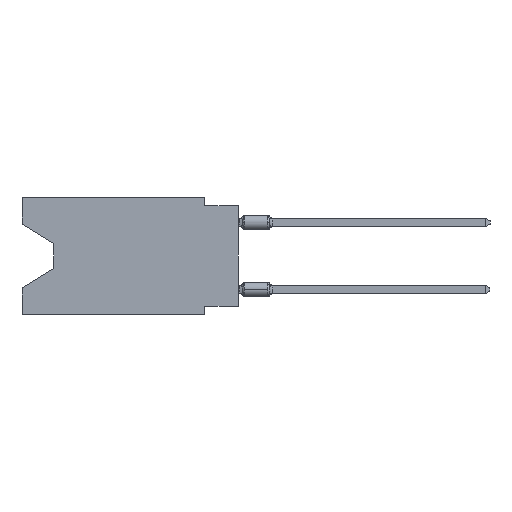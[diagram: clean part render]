
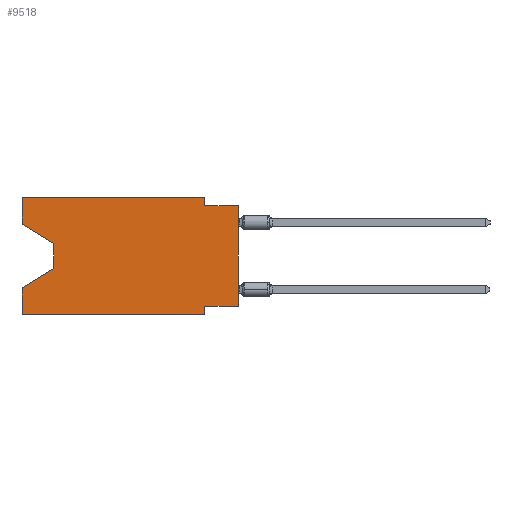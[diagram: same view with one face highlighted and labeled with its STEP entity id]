
A CAD part, left-side view. The second image highlights one B-rep face of the part: STEP entity #9518.
In plain terms, the highlighted planar face has unit normal (-1, 0, 0).
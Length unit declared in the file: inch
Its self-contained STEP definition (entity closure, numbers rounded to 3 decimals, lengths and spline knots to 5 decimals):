
#303 = CARTESIAN_POINT ( 'NONE',  ( 0., 0.55, -0.138 ) ) ;
#443 = EDGE_CURVE ( 'NONE', #11186, #7588, #18882, .T. ) ;
#929 = ORIENTED_EDGE ( 'NONE', *, *, #18731, .T. ) ;
#993 = VERTEX_POINT ( 'NONE', #1074 ) ;
#1074 = CARTESIAN_POINT ( 'NONE',  ( 0., 0.55, -0.212 ) ) ;
#1150 = DIRECTION ( 'NONE',  ( 0., 0., 1. ) ) ;
#1407 = LINE ( 'NONE', #15673, #16757 ) ;
#1430 = VERTEX_POINT ( 'NONE', #22394 ) ;
#1436 = AXIS2_PLACEMENT_3D ( 'NONE', #5542, #10573, #9273 ) ;
#1510 = EDGE_CURVE ( 'NONE', #8110, #21449, #4860, .T. ) ;
#1515 = CARTESIAN_POINT ( 'NONE',  ( 0., 0., -0.025 ) ) ;
#1518 = ORIENTED_EDGE ( 'NONE', *, *, #11480, .T. ) ;
#2066 = LINE ( 'NONE', #16099, #15612 ) ;
#2118 = VECTOR ( 'NONE', #10747, 39.37008 ) ;
#2246 = DIRECTION ( 'NONE',  ( 0., 0.855, -0.519 ) ) ;
#2607 = LINE ( 'NONE', #9733, #12410 ) ;
#2811 = DIRECTION ( 'NONE',  ( 0., 1., 0. ) ) ;
#3216 = CARTESIAN_POINT ( 'NONE',  ( 0., 0.1, 0. ) ) ;
#4379 = CARTESIAN_POINT ( 'NONE',  ( 0., 0.1, -0.325 ) ) ;
#4406 = ORIENTED_EDGE ( 'NONE', *, *, #1510, .F. ) ;
#4527 = ORIENTED_EDGE ( 'NONE', *, *, #6099, .T. ) ;
#4860 = LINE ( 'NONE', #3216, #6358 ) ;
#4877 = VERTEX_POINT ( 'NONE', #17801 ) ;
#4920 = ORIENTED_EDGE ( 'NONE', *, *, #9210, .F. ) ;
#5077 = CARTESIAN_POINT ( 'NONE',  ( 0., 0.1, -0.025 ) ) ;
#5542 = CARTESIAN_POINT ( 'NONE',  ( 0., 0.645, 0. ) ) ;
#6088 = LINE ( 'NONE', #10903, #22786 ) ;
#6099 = EDGE_CURVE ( 'NONE', #993, #4877, #6088, .T. ) ;
#6358 = VECTOR ( 'NONE', #14212, 39.37008 ) ;
#6396 = DIRECTION ( 'NONE',  ( 0., 0., -1. ) ) ;
#6989 = VECTOR ( 'NONE', #15302, 39.37008 ) ;
#7288 = CARTESIAN_POINT ( 'NONE',  ( 0., 0.645, -0.08025 ) ) ;
#7406 = FACE_OUTER_BOUND ( 'NONE', #14435, .T. ) ;
#7588 = VERTEX_POINT ( 'NONE', #12220 ) ;
#7986 = DIRECTION ( 'NONE',  ( 0., 0., 1. ) ) ;
#8110 = VERTEX_POINT ( 'NONE', #21863 ) ;
#8882 = ORIENTED_EDGE ( 'NONE', *, *, #16438, .F. ) ;
#9046 = PLANE ( 'NONE',  #1436 ) ;
#9210 = EDGE_CURVE ( 'NONE', #11186, #4877, #2066, .T. ) ;
#9273 = DIRECTION ( 'NONE',  ( 0., 0., -1. ) ) ;
#9518 = ADVANCED_FACE ( 'NONE', ( #7406 ), #9046, .F. ) ;
#9684 = ORIENTED_EDGE ( 'NONE', *, *, #15405, .F. ) ;
#9733 = CARTESIAN_POINT ( 'NONE',  ( 0., 0., 0. ) ) ;
#10573 = DIRECTION ( 'NONE',  ( 1., 0., 0. ) ) ;
#10747 = DIRECTION ( 'NONE',  ( 0., 0., -1. ) ) ;
#10903 = CARTESIAN_POINT ( 'NONE',  ( 0., 0.55, -0.212 ) ) ;
#11186 = VERTEX_POINT ( 'NONE', #22391 ) ;
#11480 = EDGE_CURVE ( 'NONE', #22761, #16186, #2607, .T. ) ;
#11852 = EDGE_CURVE ( 'NONE', #1430, #8110, #13432, .T. ) ;
#11907 = CARTESIAN_POINT ( 'NONE',  ( 0., 0.645, 0. ) ) ;
#12006 = DIRECTION ( 'NONE',  ( 0., -1., 0. ) ) ;
#12025 = CARTESIAN_POINT ( 'NONE',  ( 0., 0., -0.025 ) ) ;
#12220 = CARTESIAN_POINT ( 'NONE',  ( 0., 0.1, -0.35 ) ) ;
#12369 = ORIENTED_EDGE ( 'NONE', *, *, #17513, .T. ) ;
#12410 = VECTOR ( 'NONE', #7986, 39.37008 ) ;
#13432 = LINE ( 'NONE', #17173, #18746 ) ;
#13884 = CARTESIAN_POINT ( 'NONE',  ( 0., 0.645, -0.35 ) ) ;
#14148 = LINE ( 'NONE', #21262, #2118 ) ;
#14163 = EDGE_CURVE ( 'NONE', #21476, #1430, #17052, .T. ) ;
#14212 = DIRECTION ( 'NONE',  ( 0., 0., -1. ) ) ;
#14435 = EDGE_LOOP ( 'NONE', ( #929, #12369, #4527, #4920, #17405, #8882, #16247, #1518, #9684, #4406, #15905, #21854 ) ) ;
#15302 = DIRECTION ( 'NONE',  ( 0., -1., 0. ) ) ;
#15405 = EDGE_CURVE ( 'NONE', #21449, #16186, #22775, .T. ) ;
#15597 = VERTEX_POINT ( 'NONE', #303 ) ;
#15602 = VECTOR ( 'NONE', #12006, 39.37008 ) ;
#15612 = VECTOR ( 'NONE', #20049, 39.37008 ) ;
#15641 = LINE ( 'NONE', #22767, #23085 ) ;
#15673 = CARTESIAN_POINT ( 'NONE',  ( 0., 0., -0.325 ) ) ;
#15905 = ORIENTED_EDGE ( 'NONE', *, *, #11852, .F. ) ;
#16099 = CARTESIAN_POINT ( 'NONE',  ( 0., 0.645, 0. ) ) ;
#16186 = VERTEX_POINT ( 'NONE', #1515 ) ;
#16247 = ORIENTED_EDGE ( 'NONE', *, *, #17336, .F. ) ;
#16438 = EDGE_CURVE ( 'NONE', #17982, #7588, #15641, .T. ) ;
#16757 = VECTOR ( 'NONE', #2811, 39.37008 ) ;
#17052 = LINE ( 'NONE', #11907, #22125 ) ;
#17173 = CARTESIAN_POINT ( 'NONE',  ( 0., 0.645, 0. ) ) ;
#17241 = VECTOR ( 'NONE', #19359, 39.37008 ) ;
#17336 = EDGE_CURVE ( 'NONE', #22761, #17982, #1407, .T. ) ;
#17405 = ORIENTED_EDGE ( 'NONE', *, *, #443, .T. ) ;
#17513 = EDGE_CURVE ( 'NONE', #15597, #993, #14148, .T. ) ;
#17731 = CARTESIAN_POINT ( 'NONE',  ( 0., 0.645, -0.08025 ) ) ;
#17801 = CARTESIAN_POINT ( 'NONE',  ( 0., 0.645, -0.26975 ) ) ;
#17839 = LINE ( 'NONE', #17731, #17241 ) ;
#17982 = VERTEX_POINT ( 'NONE', #4379 ) ;
#18454 = DIRECTION ( 'NONE',  ( 0., -1., 0. ) ) ;
#18731 = EDGE_CURVE ( 'NONE', #21476, #15597, #17839, .T. ) ;
#18746 = VECTOR ( 'NONE', #18454, 39.37008 ) ;
#18882 = LINE ( 'NONE', #13884, #15602 ) ;
#19359 = DIRECTION ( 'NONE',  ( 0., -0.855, -0.519 ) ) ;
#19904 = CARTESIAN_POINT ( 'NONE',  ( 0., 0., -0.325 ) ) ;
#20049 = DIRECTION ( 'NONE',  ( 0., 0., 1. ) ) ;
#21262 = CARTESIAN_POINT ( 'NONE',  ( 0., 0.55, -0.138 ) ) ;
#21449 = VERTEX_POINT ( 'NONE', #5077 ) ;
#21476 = VERTEX_POINT ( 'NONE', #7288 ) ;
#21854 = ORIENTED_EDGE ( 'NONE', *, *, #14163, .F. ) ;
#21863 = CARTESIAN_POINT ( 'NONE',  ( 0., 0.1, 0. ) ) ;
#22125 = VECTOR ( 'NONE', #1150, 39.37008 ) ;
#22391 = CARTESIAN_POINT ( 'NONE',  ( 0., 0.645, -0.35 ) ) ;
#22394 = CARTESIAN_POINT ( 'NONE',  ( 0., 0.645, 0. ) ) ;
#22761 = VERTEX_POINT ( 'NONE', #19904 ) ;
#22767 = CARTESIAN_POINT ( 'NONE',  ( 0., 0.1, -0.35 ) ) ;
#22775 = LINE ( 'NONE', #12025, #6989 ) ;
#22786 = VECTOR ( 'NONE', #2246, 39.37008 ) ;
#23085 = VECTOR ( 'NONE', #6396, 39.37008 ) ;
